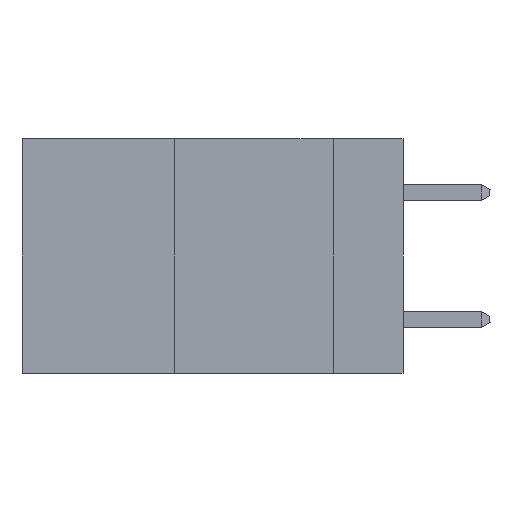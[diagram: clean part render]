
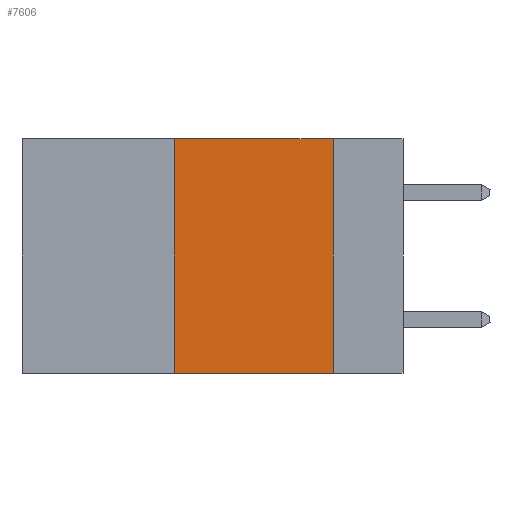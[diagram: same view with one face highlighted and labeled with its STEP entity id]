
A CAD part, left-side view. The second image highlights one B-rep face of the part: STEP entity #7606.
In plain terms, the highlighted planar face has unit normal (-1, 0, 0).
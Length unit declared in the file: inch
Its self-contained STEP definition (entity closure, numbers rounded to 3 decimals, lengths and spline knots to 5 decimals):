
#802 = VERTEX_POINT ( 'NONE', #31457 ) ;
#844 = VECTOR ( 'NONE', #22741, 39.37008 ) ;
#1050 = VERTEX_POINT ( 'NONE', #5326 ) ;
#2460 = LINE ( 'NONE', #3965, #23494 ) ;
#2947 = DIRECTION ( 'NONE',  ( 0., 0., -1. ) ) ;
#2971 = VERTEX_POINT ( 'NONE', #6014 ) ;
#3180 = EDGE_CURVE ( 'NONE', #802, #29511, #2460, .T. ) ;
#3965 = CARTESIAN_POINT ( 'NONE',  ( 0., 0.11, 0. ) ) ;
#5326 = CARTESIAN_POINT ( 'NONE',  ( 0., 0.36, 0. ) ) ;
#6014 = CARTESIAN_POINT ( 'NONE',  ( 0., 0.36, -0.37 ) ) ;
#6718 = LINE ( 'NONE', #29270, #22172 ) ;
#7606 = ADVANCED_FACE ( 'NONE', ( #29847 ), #17995, .F. ) ;
#8082 = ORIENTED_EDGE ( 'NONE', *, *, #23166, .F. ) ;
#8138 = LINE ( 'NONE', #19146, #844 ) ;
#16311 = CARTESIAN_POINT ( 'NONE',  ( 0., 0.6, 0. ) ) ;
#16482 = ORIENTED_EDGE ( 'NONE', *, *, #32136, .T. ) ;
#17995 = PLANE ( 'NONE',  #34345 ) ;
#18106 = DIRECTION ( 'NONE',  ( 0., 0., -1. ) ) ;
#19146 = CARTESIAN_POINT ( 'NONE',  ( 0., 0.36, 0. ) ) ;
#19261 = LINE ( 'NONE', #16311, #19727 ) ;
#19727 = VECTOR ( 'NONE', #22436, 39.37008 ) ;
#20772 = CARTESIAN_POINT ( 'NONE',  ( 0., 0.6, 0. ) ) ;
#21473 = EDGE_LOOP ( 'NONE', ( #25417, #8082, #35416, #16482 ) ) ;
#22172 = VECTOR ( 'NONE', #26719, 39.37008 ) ;
#22436 = DIRECTION ( 'NONE',  ( 0., -1., 0. ) ) ;
#22741 = DIRECTION ( 'NONE',  ( 0., 0., 1. ) ) ;
#22928 = EDGE_CURVE ( 'NONE', #2971, #1050, #8138, .T. ) ;
#23166 = EDGE_CURVE ( 'NONE', #1050, #802, #19261, .T. ) ;
#23494 = VECTOR ( 'NONE', #2947, 39.37008 ) ;
#25417 = ORIENTED_EDGE ( 'NONE', *, *, #3180, .F. ) ;
#26719 = DIRECTION ( 'NONE',  ( 0., -1., 0. ) ) ;
#29270 = CARTESIAN_POINT ( 'NONE',  ( 0., 0.6, -0.37 ) ) ;
#29511 = VERTEX_POINT ( 'NONE', #32157 ) ;
#29847 = FACE_OUTER_BOUND ( 'NONE', #21473, .T. ) ;
#31457 = CARTESIAN_POINT ( 'NONE',  ( 0., 0.11, 0. ) ) ;
#32136 = EDGE_CURVE ( 'NONE', #2971, #29511, #6718, .T. ) ;
#32157 = CARTESIAN_POINT ( 'NONE',  ( 0., 0.11, -0.37 ) ) ;
#34345 = AXIS2_PLACEMENT_3D ( 'NONE', #20772, #34590, #18106 ) ;
#34590 = DIRECTION ( 'NONE',  ( 1., 0., 0. ) ) ;
#35416 = ORIENTED_EDGE ( 'NONE', *, *, #22928, .F. ) ;
